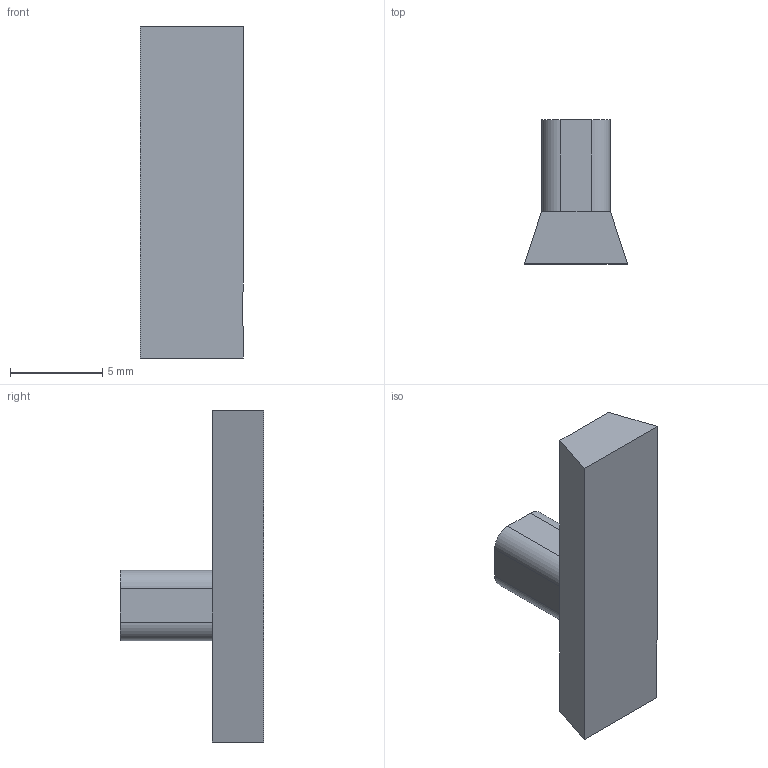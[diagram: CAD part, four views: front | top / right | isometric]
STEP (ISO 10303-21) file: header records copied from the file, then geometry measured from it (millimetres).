
FILE_DESCRIPTION((''),'2;1');
FILE_NAME('lock.stp','2013-07-01T18:24:45',('mrfr'),(''),'Autodesk Inventor 2013','Autodesk Inventor 2013','');
FILE_SCHEMA(('AUTOMOTIVE_DESIGN { 1 0 10303 214 1 1 1 1 }'));
Length unit declared in the file: millimetre
Products named in the file (1): derringer_zapadka
Bounding box: 5.6 x 7.8 x 18 mm (x, y, z)
Volume: 302 mm3; surface area: 367.1 mm2
Topology: 1 solids, 1 shells, 18 faces, 47 edges, 34 vertices
Faces by surface type: plane 14, cylinder 4
Entity records: 592 total; most frequent: CARTESIAN_POINT 97, DIRECTION 93, ORIENTED_EDGE 88, EDGE_CURVE 44, VECTOR 39, LINE 39, VERTEX_POINT 28, AXIS2_PLACEMENT_3D 27
